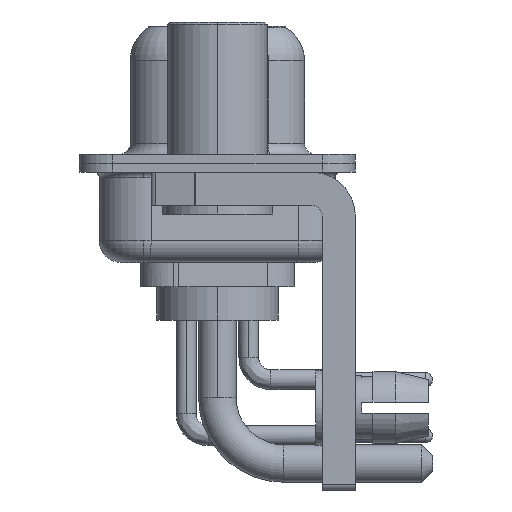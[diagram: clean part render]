
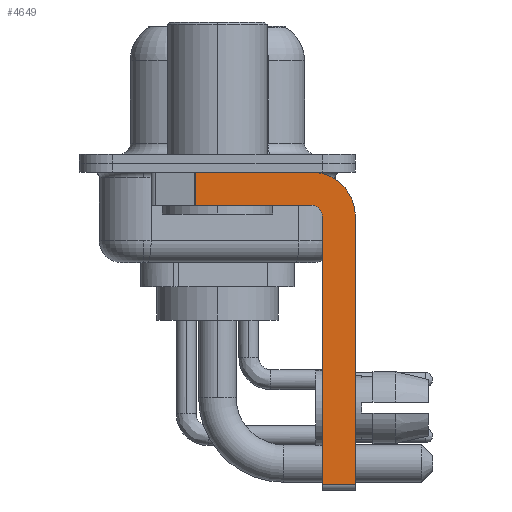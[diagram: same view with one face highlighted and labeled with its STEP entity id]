
A CAD part, left-side view. The second image highlights one B-rep face of the part: STEP entity #4649.
In plain terms, the highlighted planar face has unit normal (-1, 0, 0).
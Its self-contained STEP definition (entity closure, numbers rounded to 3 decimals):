
#192 = CIRCLE ( 'NONE', #2035, 0.5 ) ;
#355 = CARTESIAN_POINT ( 'NONE',  ( -2.9, 3., -0.4 ) ) ;
#452 = EDGE_CURVE ( 'NONE', #21904, #21906, #26616, .T. ) ;
#907 = AXIS2_PLACEMENT_3D ( 'NONE', #18036, #9024, #17747 ) ;
#1371 = DIRECTION ( 'NONE',  ( 0., 0., 1. ) ) ;
#1398 = DIRECTION ( 'NONE',  ( 0., 0., 1. ) ) ;
#2035 = AXIS2_PLACEMENT_3D ( 'NONE', #14171, #7568, #1398 ) ;
#2136 = EDGE_CURVE ( 'NONE', #24192, #26006, #192, .T. ) ;
#2322 = DIRECTION ( 'NONE',  ( 1., 0., 0. ) ) ;
#2900 = ORIENTED_EDGE ( 'NONE', *, *, #16351, .F. ) ;
#3537 = VECTOR ( 'NONE', #8378, 1000. ) ;
#4649 = ADVANCED_FACE ( 'NONE', ( #17793 ), #10955, .F. ) ;
#4688 = EDGE_CURVE ( 'NONE', #21904, #26178, #9218, .T. ) ;
#6178 = LINE ( 'NONE', #12623, #16401 ) ;
#6789 = CARTESIAN_POINT ( 'NONE',  ( -2.9, -4.25, -2.4 ) ) ;
#7157 = ORIENTED_EDGE ( 'NONE', *, *, #2136, .F. ) ;
#7568 = DIRECTION ( 'NONE',  ( -1., 0., 0. ) ) ;
#8378 = DIRECTION ( 'NONE',  ( 0., -1., 0. ) ) ;
#8455 = DIRECTION ( 'NONE',  ( 0., 1., 0. ) ) ;
#8521 = LINE ( 'NONE', #21713, #3537 ) ;
#9024 = DIRECTION ( 'NONE',  ( 1., 0., 0. ) ) ;
#9218 = LINE ( 'NONE', #15387, #25627 ) ;
#9462 = ORIENTED_EDGE ( 'NONE', *, *, #4688, .T. ) ;
#10275 = VECTOR ( 'NONE', #16542, 1000. ) ;
#10466 = VERTEX_POINT ( 'NONE', #14697 ) ;
#10542 = CIRCLE ( 'NONE', #907, 2. ) ;
#10955 = PLANE ( 'NONE',  #19198 ) ;
#12176 = EDGE_CURVE ( 'NONE', #25096, #21215, #8521, .T. ) ;
#12623 = CARTESIAN_POINT ( 'NONE',  ( -2.9, -4.25, -1.9 ) ) ;
#12992 = VECTOR ( 'NONE', #1371, 1000. ) ;
#13057 = EDGE_CURVE ( 'NONE', #26006, #26178, #6178, .T. ) ;
#13627 = ORIENTED_EDGE ( 'NONE', *, *, #27085, .F. ) ;
#14171 = CARTESIAN_POINT ( 'NONE',  ( -2.9, -4.25, -2.4 ) ) ;
#14697 = CARTESIAN_POINT ( 'NONE',  ( -2.9, -6.25, -2.4 ) ) ;
#15387 = CARTESIAN_POINT ( 'NONE',  ( -2.9, 0.978, -1.9 ) ) ;
#16351 = EDGE_CURVE ( 'NONE', #21906, #10466, #10542, .T. ) ;
#16401 = VECTOR ( 'NONE', #8455, 1000. ) ;
#16513 = CARTESIAN_POINT ( 'NONE',  ( -2.9, 0.978, -0.4 ) ) ;
#16542 = DIRECTION ( 'NONE',  ( 0., 0., -1. ) ) ;
#17368 = CARTESIAN_POINT ( 'NONE',  ( -2.9, -4.25, -1.9 ) ) ;
#17638 = CARTESIAN_POINT ( 'NONE',  ( -2.9, 0.978, -1.9 ) ) ;
#17747 = DIRECTION ( 'NONE',  ( 0., 0., -1. ) ) ;
#17793 = FACE_OUTER_BOUND ( 'NONE', #26822, .T. ) ;
#18036 = CARTESIAN_POINT ( 'NONE',  ( -2.9, -4.25, -2.4 ) ) ;
#18390 = CARTESIAN_POINT ( 'NONE',  ( -2.9, -6.25, -2.4 ) ) ;
#19198 = AXIS2_PLACEMENT_3D ( 'NONE', #6789, #2322, #26148 ) ;
#19452 = CARTESIAN_POINT ( 'NONE',  ( -2.9, -4.75, -14.55 ) ) ;
#19707 = ORIENTED_EDGE ( 'NONE', *, *, #452, .F. ) ;
#20277 = DIRECTION ( 'NONE',  ( 0., -1., 0. ) ) ;
#20394 = CARTESIAN_POINT ( 'NONE',  ( -2.9, -6.25, -14.55 ) ) ;
#21215 = VERTEX_POINT ( 'NONE', #20394 ) ;
#21713 = CARTESIAN_POINT ( 'NONE',  ( -2.9, -4.25, -14.55 ) ) ;
#21904 = VERTEX_POINT ( 'NONE', #16513 ) ;
#21906 = VERTEX_POINT ( 'NONE', #23244 ) ;
#22091 = ORIENTED_EDGE ( 'NONE', *, *, #25288, .F. ) ;
#22284 = LINE ( 'NONE', #18390, #10275 ) ;
#22577 = CARTESIAN_POINT ( 'NONE',  ( -2.9, -4.75, -2.4 ) ) ;
#23027 = LINE ( 'NONE', #24908, #12992 ) ;
#23244 = CARTESIAN_POINT ( 'NONE',  ( -2.9, -4.25, -0.4 ) ) ;
#24137 = DIRECTION ( 'NONE',  ( 0., 0., -1. ) ) ;
#24192 = VERTEX_POINT ( 'NONE', #22577 ) ;
#24376 = ORIENTED_EDGE ( 'NONE', *, *, #13057, .F. ) ;
#24908 = CARTESIAN_POINT ( 'NONE',  ( -2.9, -4.75, -14.8 ) ) ;
#25096 = VERTEX_POINT ( 'NONE', #19452 ) ;
#25288 = EDGE_CURVE ( 'NONE', #25096, #24192, #23027, .T. ) ;
#25396 = VECTOR ( 'NONE', #20277, 1000. ) ;
#25627 = VECTOR ( 'NONE', #24137, 1000. ) ;
#26006 = VERTEX_POINT ( 'NONE', #17368 ) ;
#26148 = DIRECTION ( 'NONE',  ( 0., 0., -1. ) ) ;
#26178 = VERTEX_POINT ( 'NONE', #17638 ) ;
#26616 = LINE ( 'NONE', #355, #25396 ) ;
#26822 = EDGE_LOOP ( 'NONE', ( #19707, #9462, #24376, #7157, #22091, #27923, #13627, #2900 ) ) ;
#27085 = EDGE_CURVE ( 'NONE', #10466, #21215, #22284, .T. ) ;
#27923 = ORIENTED_EDGE ( 'NONE', *, *, #12176, .T. ) ;
